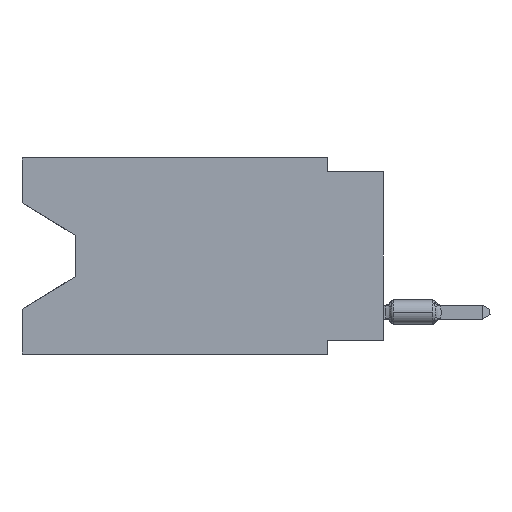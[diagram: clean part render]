
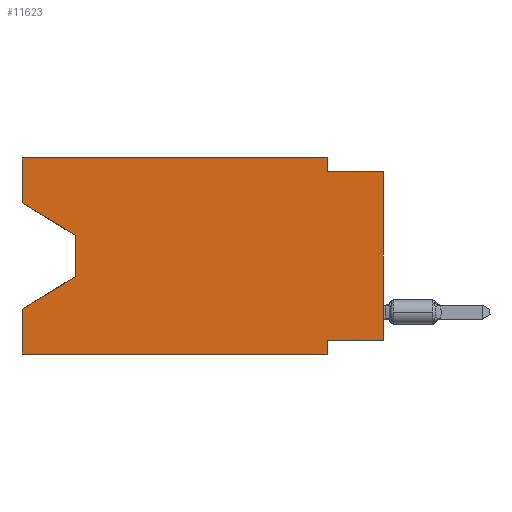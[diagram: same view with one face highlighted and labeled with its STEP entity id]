
A CAD part, left-side view. The second image highlights one B-rep face of the part: STEP entity #11623.
In plain terms, the highlighted planar face has unit normal (-1, 0, 0).
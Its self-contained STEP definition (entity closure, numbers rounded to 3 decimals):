
#164 = ORIENTED_EDGE ( 'NONE', *, *, #14007, .F. ) ;
#207 = ORIENTED_EDGE ( 'NONE', *, *, #8263, .T. ) ;
#265 = ORIENTED_EDGE ( 'NONE', *, *, #11347, .F. ) ;
#335 = DIRECTION ( 'NONE',  ( 0., 0., 1. ) ) ;
#1150 = VECTOR ( 'NONE', #4024, 1000. ) ;
#1518 = LINE ( 'NONE', #5970, #6760 ) ;
#1562 = VECTOR ( 'NONE', #20288, 1000. ) ;
#1621 = LINE ( 'NONE', #12700, #10153 ) ;
#1821 = VERTEX_POINT ( 'NONE', #11606 ) ;
#2356 = LINE ( 'NONE', #22657, #8220 ) ;
#2522 = DIRECTION ( 'NONE',  ( 1., 0., 0. ) ) ;
#2678 = EDGE_CURVE ( 'NONE', #13900, #19183, #20505, .T. ) ;
#3085 = VERTEX_POINT ( 'NONE', #22729 ) ;
#3100 = EDGE_CURVE ( 'NONE', #19183, #3085, #4241, .T. ) ;
#3610 = LINE ( 'NONE', #27663, #17112 ) ;
#3635 = VERTEX_POINT ( 'NONE', #16375 ) ;
#4024 = DIRECTION ( 'NONE',  ( 0., -1., 0. ) ) ;
#4102 = CARTESIAN_POINT ( 'NONE',  ( 0., 13.97, -3.505 ) ) ;
#4241 = LINE ( 'NONE', #14647, #22302 ) ;
#4250 = ORIENTED_EDGE ( 'NONE', *, *, #5718, .T. ) ;
#5079 = DIRECTION ( 'NONE',  ( 0., 0.855, -0.519 ) ) ;
#5328 = VECTOR ( 'NONE', #23325, 1000. ) ;
#5487 = EDGE_CURVE ( 'NONE', #13900, #12021, #2356, .T. ) ;
#5718 = EDGE_CURVE ( 'NONE', #25476, #15211, #1621, .T. ) ;
#5862 = ORIENTED_EDGE ( 'NONE', *, *, #21060, .F. ) ;
#5921 = CARTESIAN_POINT ( 'NONE',  ( 0., 13.97, -5.385 ) ) ;
#5970 = CARTESIAN_POINT ( 'NONE',  ( 0., 16.383, 0. ) ) ;
#6024 = LINE ( 'NONE', #8318, #25066 ) ;
#6100 = DIRECTION ( 'NONE',  ( 0., 0., -1. ) ) ;
#6315 = LINE ( 'NONE', #15113, #1150 ) ;
#6557 = VERTEX_POINT ( 'NONE', #28301 ) ;
#6760 = VECTOR ( 'NONE', #28028, 1000. ) ;
#8220 = VECTOR ( 'NONE', #335, 1000. ) ;
#8257 = CARTESIAN_POINT ( 'NONE',  ( 0., 2.54, 0. ) ) ;
#8263 = EDGE_CURVE ( 'NONE', #23810, #6557, #17784, .T. ) ;
#8318 = CARTESIAN_POINT ( 'NONE',  ( 0., 13.97, -3.505 ) ) ;
#8395 = VERTEX_POINT ( 'NONE', #19065 ) ;
#8645 = DIRECTION ( 'NONE',  ( 0., -0.855, -0.519 ) ) ;
#8877 = EDGE_CURVE ( 'NONE', #8395, #3085, #3610, .T. ) ;
#9504 = VECTOR ( 'NONE', #6100, 1000. ) ;
#9529 = CARTESIAN_POINT ( 'NONE',  ( 0., 0., -8.255 ) ) ;
#9865 = ORIENTED_EDGE ( 'NONE', *, *, #19621, .T. ) ;
#10005 = ORIENTED_EDGE ( 'NONE', *, *, #2678, .F. ) ;
#10153 = VECTOR ( 'NONE', #8645, 1000. ) ;
#10788 = DIRECTION ( 'NONE',  ( 0., 0., -1. ) ) ;
#10966 = CARTESIAN_POINT ( 'NONE',  ( 0., 2.54, -8.255 ) ) ;
#11347 = EDGE_CURVE ( 'NONE', #25476, #3635, #1518, .T. ) ;
#11403 = CARTESIAN_POINT ( 'NONE',  ( 0., 0., -0.635 ) ) ;
#11606 = CARTESIAN_POINT ( 'NONE',  ( 0., 2.54, -0.635 ) ) ;
#11623 = ADVANCED_FACE ( 'NONE', ( #22826 ), #14024, .F. ) ;
#11860 = CARTESIAN_POINT ( 'NONE',  ( 0., 16.383, 0. ) ) ;
#12021 = VERTEX_POINT ( 'NONE', #11403 ) ;
#12212 = ORIENTED_EDGE ( 'NONE', *, *, #5487, .T. ) ;
#12217 = ORIENTED_EDGE ( 'NONE', *, *, #8877, .T. ) ;
#12700 = CARTESIAN_POINT ( 'NONE',  ( 0., 16.383, -2.038 ) ) ;
#13138 = ORIENTED_EDGE ( 'NONE', *, *, #19647, .F. ) ;
#13370 = ORIENTED_EDGE ( 'NONE', *, *, #3100, .F. ) ;
#13900 = VERTEX_POINT ( 'NONE', #23469 ) ;
#14007 = EDGE_CURVE ( 'NONE', #8395, #6557, #26331, .T. ) ;
#14024 = PLANE ( 'NONE',  #19619 ) ;
#14224 = CARTESIAN_POINT ( 'NONE',  ( 0., 0., -0.635 ) ) ;
#14647 = CARTESIAN_POINT ( 'NONE',  ( 0., 2.54, -8.89 ) ) ;
#15049 = VECTOR ( 'NONE', #5079, 1000. ) ;
#15113 = CARTESIAN_POINT ( 'NONE',  ( 0., 16.383, 0. ) ) ;
#15211 = VERTEX_POINT ( 'NONE', #4102 ) ;
#16283 = DIRECTION ( 'NONE',  ( 0., -1., 0. ) ) ;
#16375 = CARTESIAN_POINT ( 'NONE',  ( 0., 16.383, 0. ) ) ;
#17112 = VECTOR ( 'NONE', #16283, 1000. ) ;
#17784 = LINE ( 'NONE', #24701, #15049 ) ;
#19065 = CARTESIAN_POINT ( 'NONE',  ( 0., 16.383, -8.89 ) ) ;
#19183 = VERTEX_POINT ( 'NONE', #10966 ) ;
#19245 = LINE ( 'NONE', #8257, #9504 ) ;
#19246 = VERTEX_POINT ( 'NONE', #21504 ) ;
#19619 = AXIS2_PLACEMENT_3D ( 'NONE', #11860, #2522, #20111 ) ;
#19621 = EDGE_CURVE ( 'NONE', #15211, #23810, #6024, .T. ) ;
#19647 = EDGE_CURVE ( 'NONE', #3635, #19246, #6315, .T. ) ;
#20111 = DIRECTION ( 'NONE',  ( 0., 0., -1. ) ) ;
#20288 = DIRECTION ( 'NONE',  ( 0., 0., 1. ) ) ;
#20505 = LINE ( 'NONE', #9529, #26429 ) ;
#21060 = EDGE_CURVE ( 'NONE', #1821, #12021, #25192, .T. ) ;
#21504 = CARTESIAN_POINT ( 'NONE',  ( 0., 2.54, 0. ) ) ;
#21687 = EDGE_CURVE ( 'NONE', #19246, #1821, #19245, .T. ) ;
#22038 = CARTESIAN_POINT ( 'NONE',  ( 0., 16.383, -2.038 ) ) ;
#22302 = VECTOR ( 'NONE', #23442, 1000. ) ;
#22657 = CARTESIAN_POINT ( 'NONE',  ( 0., 0., 0. ) ) ;
#22729 = CARTESIAN_POINT ( 'NONE',  ( 0., 2.54, -8.89 ) ) ;
#22826 = FACE_OUTER_BOUND ( 'NONE', #23393, .T. ) ;
#23325 = DIRECTION ( 'NONE',  ( 0., -1., 0. ) ) ;
#23393 = EDGE_LOOP ( 'NONE', ( #4250, #9865, #207, #164, #12217, #13370, #10005, #12212, #5862, #25726, #13138, #265 ) ) ;
#23442 = DIRECTION ( 'NONE',  ( 0., 0., -1. ) ) ;
#23469 = CARTESIAN_POINT ( 'NONE',  ( 0., 0., -8.255 ) ) ;
#23810 = VERTEX_POINT ( 'NONE', #5921 ) ;
#24182 = CARTESIAN_POINT ( 'NONE',  ( 0., 16.383, 0. ) ) ;
#24701 = CARTESIAN_POINT ( 'NONE',  ( 0., 13.97, -5.385 ) ) ;
#25066 = VECTOR ( 'NONE', #10788, 1000. ) ;
#25192 = LINE ( 'NONE', #14224, #5328 ) ;
#25476 = VERTEX_POINT ( 'NONE', #22038 ) ;
#25726 = ORIENTED_EDGE ( 'NONE', *, *, #21687, .F. ) ;
#26331 = LINE ( 'NONE', #24182, #1562 ) ;
#26429 = VECTOR ( 'NONE', #27116, 1000. ) ;
#27116 = DIRECTION ( 'NONE',  ( 0., 1., 0. ) ) ;
#27663 = CARTESIAN_POINT ( 'NONE',  ( 0., 16.383, -8.89 ) ) ;
#28028 = DIRECTION ( 'NONE',  ( 0., 0., 1. ) ) ;
#28301 = CARTESIAN_POINT ( 'NONE',  ( 0., 16.383, -6.852 ) ) ;
